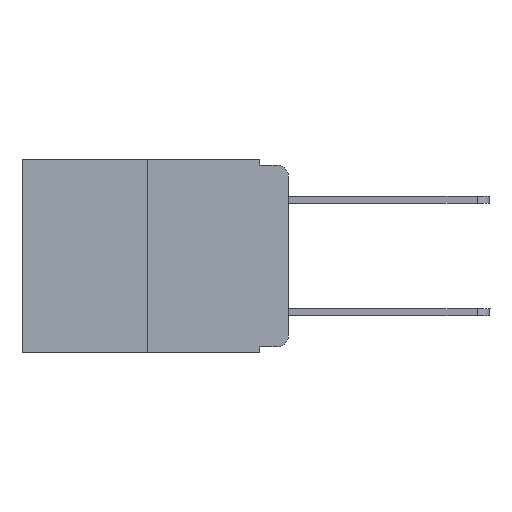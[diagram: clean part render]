
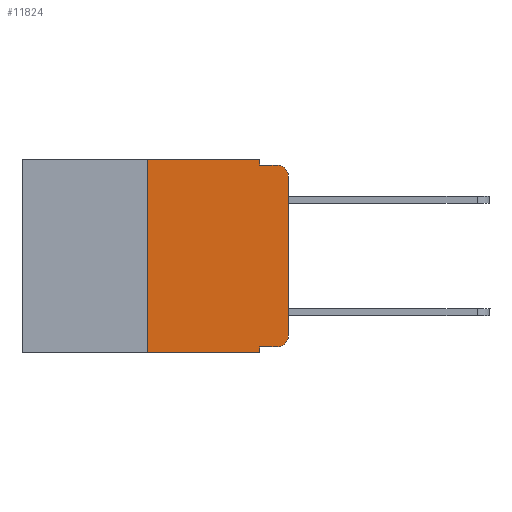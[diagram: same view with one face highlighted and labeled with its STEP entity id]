
A CAD part, left-side view. The second image highlights one B-rep face of the part: STEP entity #11824.
In plain terms, the highlighted planar face has unit normal (-1, 0, 0).
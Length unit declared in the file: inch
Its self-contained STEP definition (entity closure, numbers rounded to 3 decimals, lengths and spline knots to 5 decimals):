
#13 = ORIENTED_EDGE ( 'NONE', *, *, #4892, .T. ) ;
#31 = CARTESIAN_POINT ( 'NONE',  ( 0., 0.25, 0. ) ) ;
#290 = DIRECTION ( 'NONE',  ( -1., 0., 0. ) ) ;
#304 = VERTEX_POINT ( 'NONE', #6679 ) ;
#396 = EDGE_LOOP ( 'NONE', ( #14247, #1681, #3310, #2690, #4275, #11830, #13, #12313, #6735, #1089 ) ) ;
#639 = DIRECTION ( 'NONE',  ( 0., 0., -1. ) ) ;
#1089 = ORIENTED_EDGE ( 'NONE', *, *, #5731, .T. ) ;
#1207 = VERTEX_POINT ( 'NONE', #8151 ) ;
#1263 = CARTESIAN_POINT ( 'NONE',  ( 0., 0.473, 0. ) ) ;
#1271 = VERTEX_POINT ( 'NONE', #1703 ) ;
#1272 = DIRECTION ( 'NONE',  ( 0., 0., 1. ) ) ;
#1344 = LINE ( 'NONE', #31, #3547 ) ;
#1681 = ORIENTED_EDGE ( 'NONE', *, *, #3084, .T. ) ;
#1703 = CARTESIAN_POINT ( 'NONE',  ( 0., 0.051, -0.343 ) ) ;
#1709 = PLANE ( 'NONE',  #10177 ) ;
#2008 = VERTEX_POINT ( 'NONE', #11256 ) ;
#2051 = EDGE_CURVE ( 'NONE', #11762, #7105, #11183, .T. ) ;
#2260 = VECTOR ( 'NONE', #13762, 39.37008 ) ;
#2372 = CARTESIAN_POINT ( 'NONE',  ( 0., 0.051, -0.01 ) ) ;
#2386 = VECTOR ( 'NONE', #3209, 39.37008 ) ;
#2690 = ORIENTED_EDGE ( 'NONE', *, *, #4492, .F. ) ;
#2716 = CARTESIAN_POINT ( 'NONE',  ( 0., 0.051, -0.333 ) ) ;
#2720 = EDGE_CURVE ( 'NONE', #12961, #14028, #8042, .T. ) ;
#2855 = VECTOR ( 'NONE', #10512, 39.37008 ) ;
#2891 = DIRECTION ( 'NONE',  ( 0., -1., 0. ) ) ;
#3084 = EDGE_CURVE ( 'NONE', #1207, #7824, #14227, .T. ) ;
#3209 = DIRECTION ( 'NONE',  ( 0., 0., -1. ) ) ;
#3310 = ORIENTED_EDGE ( 'NONE', *, *, #8406, .F. ) ;
#3547 = VECTOR ( 'NONE', #1272, 39.37008 ) ;
#3586 = LINE ( 'NONE', #5907, #5454 ) ;
#3905 = CARTESIAN_POINT ( 'NONE',  ( 0., 0.02, -0.333 ) ) ;
#4275 = ORIENTED_EDGE ( 'NONE', *, *, #2051, .F. ) ;
#4284 = DIRECTION ( 'NONE',  ( -1., 0., 0. ) ) ;
#4492 = EDGE_CURVE ( 'NONE', #7105, #12947, #9418, .T. ) ;
#4892 = EDGE_CURVE ( 'NONE', #2008, #1271, #3586, .T. ) ;
#5110 = CARTESIAN_POINT ( 'NONE',  ( 0., 0.051, -0.01 ) ) ;
#5454 = VECTOR ( 'NONE', #6112, 39.37008 ) ;
#5601 = VECTOR ( 'NONE', #5793, 39.37008 ) ;
#5634 = DIRECTION ( 'NONE',  ( 0., 0., -1. ) ) ;
#5731 = EDGE_CURVE ( 'NONE', #14028, #304, #11044, .T. ) ;
#5793 = DIRECTION ( 'NONE',  ( 0., -1., 0. ) ) ;
#5907 = CARTESIAN_POINT ( 'NONE',  ( 0., 0.473, -0.343 ) ) ;
#6112 = DIRECTION ( 'NONE',  ( 0., -1., 0. ) ) ;
#6119 = CARTESIAN_POINT ( 'NONE',  ( 0., 0.473, 0. ) ) ;
#6134 = VECTOR ( 'NONE', #7289, 39.37008 ) ;
#6295 = EDGE_CURVE ( 'NONE', #304, #1207, #10360, .T. ) ;
#6679 = CARTESIAN_POINT ( 'NONE',  ( 0., 0., -0.313 ) ) ;
#6735 = ORIENTED_EDGE ( 'NONE', *, *, #2720, .T. ) ;
#7105 = VERTEX_POINT ( 'NONE', #9482 ) ;
#7289 = DIRECTION ( 'NONE',  ( 0., 0., -1. ) ) ;
#7556 = AXIS2_PLACEMENT_3D ( 'NONE', #8931, #4284, #13228 ) ;
#7824 = VERTEX_POINT ( 'NONE', #12255 ) ;
#8042 = LINE ( 'NONE', #11323, #5601 ) ;
#8151 = CARTESIAN_POINT ( 'NONE',  ( 0., 0., -0.03 ) ) ;
#8155 = CARTESIAN_POINT ( 'NONE',  ( 0., 0., 0. ) ) ;
#8406 = EDGE_CURVE ( 'NONE', #12947, #7824, #12605, .T. ) ;
#8566 = CARTESIAN_POINT ( 'NONE',  ( 0., 0.051, 0. ) ) ;
#8931 = CARTESIAN_POINT ( 'NONE',  ( 0., 0.02, -0.313 ) ) ;
#9418 = LINE ( 'NONE', #12611, #6134 ) ;
#9477 = FACE_OUTER_BOUND ( 'NONE', #396, .T. ) ;
#9482 = CARTESIAN_POINT ( 'NONE',  ( 0., 0.051, 0. ) ) ;
#9606 = LINE ( 'NONE', #8566, #2386 ) ;
#10032 = AXIS2_PLACEMENT_3D ( 'NONE', #12109, #290, #5634 ) ;
#10177 = AXIS2_PLACEMENT_3D ( 'NONE', #6119, #10581, #639 ) ;
#10360 = LINE ( 'NONE', #8155, #2260 ) ;
#10512 = DIRECTION ( 'NONE',  ( 0., -1., 0. ) ) ;
#10581 = DIRECTION ( 'NONE',  ( 1., 0., 0. ) ) ;
#11044 = CIRCLE ( 'NONE', #7556, 0.02 ) ;
#11183 = LINE ( 'NONE', #1263, #11619 ) ;
#11256 = CARTESIAN_POINT ( 'NONE',  ( 0., 0.25, -0.343 ) ) ;
#11323 = CARTESIAN_POINT ( 'NONE',  ( 0., 0.051, -0.333 ) ) ;
#11511 = CARTESIAN_POINT ( 'NONE',  ( 0., 0.25, 0. ) ) ;
#11619 = VECTOR ( 'NONE', #2891, 39.37008 ) ;
#11762 = VERTEX_POINT ( 'NONE', #11511 ) ;
#11824 = ADVANCED_FACE ( 'NONE', ( #9477 ), #1709, .F. ) ;
#11830 = ORIENTED_EDGE ( 'NONE', *, *, #13846, .F. ) ;
#12109 = CARTESIAN_POINT ( 'NONE',  ( 0., 0.02, -0.03 ) ) ;
#12255 = CARTESIAN_POINT ( 'NONE',  ( 0., 0.02, -0.01 ) ) ;
#12313 = ORIENTED_EDGE ( 'NONE', *, *, #13651, .F. ) ;
#12605 = LINE ( 'NONE', #5110, #2855 ) ;
#12611 = CARTESIAN_POINT ( 'NONE',  ( 0., 0.051, 0. ) ) ;
#12947 = VERTEX_POINT ( 'NONE', #2372 ) ;
#12961 = VERTEX_POINT ( 'NONE', #2716 ) ;
#13228 = DIRECTION ( 'NONE',  ( 0., 0., -1. ) ) ;
#13651 = EDGE_CURVE ( 'NONE', #12961, #1271, #9606, .T. ) ;
#13762 = DIRECTION ( 'NONE',  ( 0., 0., 1. ) ) ;
#13846 = EDGE_CURVE ( 'NONE', #2008, #11762, #1344, .T. ) ;
#14028 = VERTEX_POINT ( 'NONE', #3905 ) ;
#14227 = CIRCLE ( 'NONE', #10032, 0.02 ) ;
#14247 = ORIENTED_EDGE ( 'NONE', *, *, #6295, .T. ) ;
